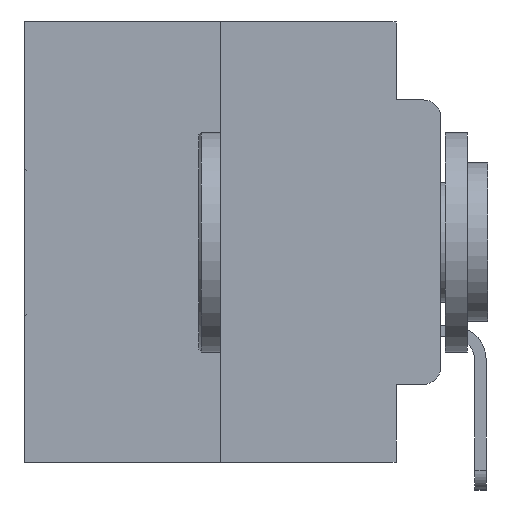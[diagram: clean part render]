
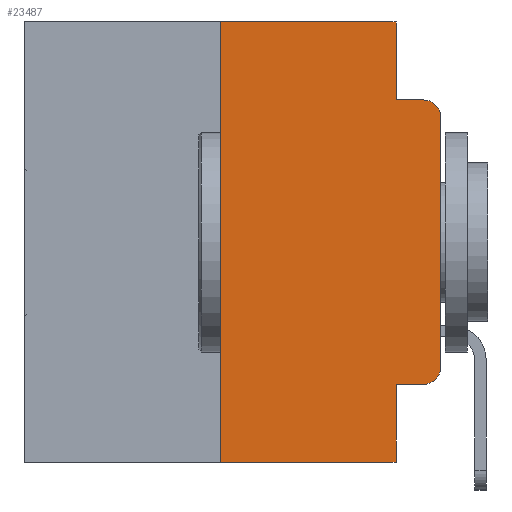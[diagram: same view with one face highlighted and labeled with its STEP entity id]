
A CAD part, left-side view. The second image highlights one B-rep face of the part: STEP entity #23487.
In plain terms, the highlighted planar face has unit normal (-1, 0, 0).
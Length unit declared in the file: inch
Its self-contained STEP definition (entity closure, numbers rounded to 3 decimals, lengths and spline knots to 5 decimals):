
#5 = DIRECTION ( 'NONE',  ( 1., 0., 0. ) ) ;
#394 = CARTESIAN_POINT ( 'NONE',  ( 0., 0.02, -0.3915 ) ) ;
#516 = VERTEX_POINT ( 'NONE', #8817 ) ;
#640 = VECTOR ( 'NONE', #2313, 39.37008 ) ;
#953 = EDGE_CURVE ( 'NONE', #17393, #27465, #20028, .T. ) ;
#1070 = DIRECTION ( 'NONE',  ( 0., 0., -1. ) ) ;
#1185 = VECTOR ( 'NONE', #14962, 39.37008 ) ;
#1536 = DIRECTION ( 'NONE',  ( 0., -1., 0. ) ) ;
#2313 = DIRECTION ( 'NONE',  ( 0., 0., -1. ) ) ;
#2385 = CARTESIAN_POINT ( 'NONE',  ( 0., 0.473, 0. ) ) ;
#2426 = LINE ( 'NONE', #26093, #11518 ) ;
#2610 = FACE_OUTER_BOUND ( 'NONE', #7854, .T. ) ;
#2640 = EDGE_CURVE ( 'NONE', #13239, #7189, #5625, .T. ) ;
#3439 = VECTOR ( 'NONE', #26139, 39.37008 ) ;
#4262 = PLANE ( 'NONE',  #7263 ) ;
#4291 = EDGE_CURVE ( 'NONE', #7189, #12286, #26947, .T. ) ;
#4445 = AXIS2_PLACEMENT_3D ( 'NONE', #394, #18417, #18715 ) ;
#4476 = VECTOR ( 'NONE', #18218, 39.37008 ) ;
#5040 = ORIENTED_EDGE ( 'NONE', *, *, #953, .T. ) ;
#5625 = LINE ( 'NONE', #9272, #19716 ) ;
#7120 = ORIENTED_EDGE ( 'NONE', *, *, #26117, .T. ) ;
#7143 = DIRECTION ( 'NONE',  ( 0., -1., 0. ) ) ;
#7189 = VERTEX_POINT ( 'NONE', #20800 ) ;
#7263 = AXIS2_PLACEMENT_3D ( 'NONE', #2385, #5, #15454 ) ;
#7296 = CARTESIAN_POINT ( 'NONE',  ( 0., 0.25, 0. ) ) ;
#7625 = CARTESIAN_POINT ( 'NONE',  ( 0., 0.473, -0.5 ) ) ;
#7854 = EDGE_LOOP ( 'NONE', ( #26755, #7120, #21348, #14099, #8255, #10530, #15684, #24738, #5040, #23492 ) ) ;
#8255 = ORIENTED_EDGE ( 'NONE', *, *, #2640, .F. ) ;
#8698 = CARTESIAN_POINT ( 'NONE',  ( 0., 0.02, -0.0885 ) ) ;
#8817 = CARTESIAN_POINT ( 'NONE',  ( 0., 0.051, -0.5 ) ) ;
#8873 = EDGE_CURVE ( 'NONE', #13942, #12362, #2426, .T. ) ;
#9090 = CARTESIAN_POINT ( 'NONE',  ( 0., 0.051, 0. ) ) ;
#9272 = CARTESIAN_POINT ( 'NONE',  ( 0., 0.473, 0. ) ) ;
#9791 = CARTESIAN_POINT ( 'NONE',  ( 0., 0.02, -0.4115 ) ) ;
#10530 = ORIENTED_EDGE ( 'NONE', *, *, #19715, .F. ) ;
#11140 = CARTESIAN_POINT ( 'NONE',  ( 0., 0.051, -0.0885 ) ) ;
#11518 = VECTOR ( 'NONE', #12609, 39.37008 ) ;
#12065 = DIRECTION ( 'NONE',  ( -1., 0., 0. ) ) ;
#12168 = CARTESIAN_POINT ( 'NONE',  ( 0., 0.02, -0.1085 ) ) ;
#12286 = VERTEX_POINT ( 'NONE', #21158 ) ;
#12362 = VERTEX_POINT ( 'NONE', #19411 ) ;
#12609 = DIRECTION ( 'NONE',  ( 0., 0., 1. ) ) ;
#13239 = VERTEX_POINT ( 'NONE', #18479 ) ;
#13701 = EDGE_CURVE ( 'NONE', #16897, #516, #19521, .T. ) ;
#13942 = VERTEX_POINT ( 'NONE', #20642 ) ;
#14033 = CIRCLE ( 'NONE', #24288, 0.02 ) ;
#14046 = EDGE_CURVE ( 'NONE', #27465, #13942, #27276, .T. ) ;
#14099 = ORIENTED_EDGE ( 'NONE', *, *, #4291, .F. ) ;
#14579 = LINE ( 'NONE', #11140, #20922 ) ;
#14962 = DIRECTION ( 'NONE',  ( 0., -1., 0. ) ) ;
#15022 = LINE ( 'NONE', #7296, #3439 ) ;
#15454 = DIRECTION ( 'NONE',  ( 0., 0., -1. ) ) ;
#15684 = ORIENTED_EDGE ( 'NONE', *, *, #13701, .T. ) ;
#15753 = CARTESIAN_POINT ( 'NONE',  ( 0., 0.051, 0. ) ) ;
#15934 = CARTESIAN_POINT ( 'NONE',  ( 0., 0.25, -0.5 ) ) ;
#16222 = CARTESIAN_POINT ( 'NONE',  ( 0., 0.051, -0.4115 ) ) ;
#16897 = VERTEX_POINT ( 'NONE', #15934 ) ;
#17393 = VERTEX_POINT ( 'NONE', #16222 ) ;
#18218 = DIRECTION ( 'NONE',  ( 0., 0., -1. ) ) ;
#18417 = DIRECTION ( 'NONE',  ( -1., 0., 0. ) ) ;
#18479 = CARTESIAN_POINT ( 'NONE',  ( 0., 0.25, 0. ) ) ;
#18715 = DIRECTION ( 'NONE',  ( 0., 0., -1. ) ) ;
#18778 = EDGE_CURVE ( 'NONE', #17393, #516, #22494, .T. ) ;
#19411 = CARTESIAN_POINT ( 'NONE',  ( 0., 0., -0.1085 ) ) ;
#19521 = LINE ( 'NONE', #7625, #1185 ) ;
#19715 = EDGE_CURVE ( 'NONE', #16897, #13239, #15022, .T. ) ;
#19716 = VECTOR ( 'NONE', #7143, 39.37008 ) ;
#20028 = LINE ( 'NONE', #21685, #27348 ) ;
#20642 = CARTESIAN_POINT ( 'NONE',  ( 0., 0., -0.3915 ) ) ;
#20800 = CARTESIAN_POINT ( 'NONE',  ( 0., 0.051, 0. ) ) ;
#20922 = VECTOR ( 'NONE', #29027, 39.37008 ) ;
#21158 = CARTESIAN_POINT ( 'NONE',  ( 0., 0.051, -0.0885 ) ) ;
#21348 = ORIENTED_EDGE ( 'NONE', *, *, #27796, .F. ) ;
#21685 = CARTESIAN_POINT ( 'NONE',  ( 0., 0.051, -0.4115 ) ) ;
#22494 = LINE ( 'NONE', #15753, #640 ) ;
#23487 = ADVANCED_FACE ( 'NONE', ( #2610 ), #4262, .F. ) ;
#23492 = ORIENTED_EDGE ( 'NONE', *, *, #14046, .T. ) ;
#24288 = AXIS2_PLACEMENT_3D ( 'NONE', #12168, #12065, #1070 ) ;
#24738 = ORIENTED_EDGE ( 'NONE', *, *, #18778, .F. ) ;
#26093 = CARTESIAN_POINT ( 'NONE',  ( 0., 0., 0. ) ) ;
#26117 = EDGE_CURVE ( 'NONE', #12362, #28199, #14033, .T. ) ;
#26139 = DIRECTION ( 'NONE',  ( 0., 0., 1. ) ) ;
#26755 = ORIENTED_EDGE ( 'NONE', *, *, #8873, .T. ) ;
#26947 = LINE ( 'NONE', #9090, #4476 ) ;
#27276 = CIRCLE ( 'NONE', #4445, 0.02 ) ;
#27348 = VECTOR ( 'NONE', #1536, 39.37008 ) ;
#27465 = VERTEX_POINT ( 'NONE', #9791 ) ;
#27796 = EDGE_CURVE ( 'NONE', #12286, #28199, #14579, .T. ) ;
#28199 = VERTEX_POINT ( 'NONE', #8698 ) ;
#29027 = DIRECTION ( 'NONE',  ( 0., -1., 0. ) ) ;
